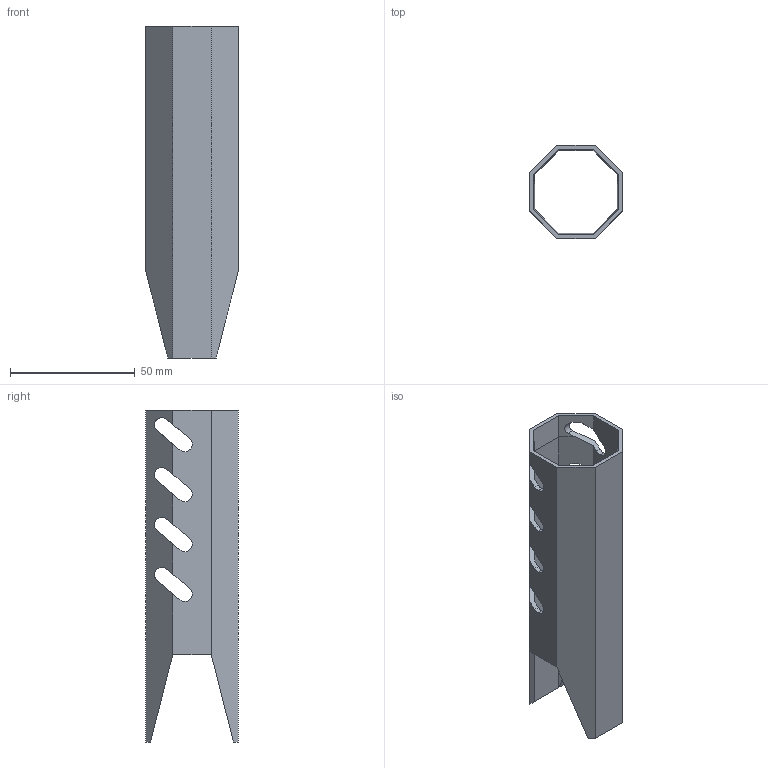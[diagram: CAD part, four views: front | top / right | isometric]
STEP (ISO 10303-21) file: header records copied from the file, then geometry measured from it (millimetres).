
FILE_DESCRIPTION (( 'STEP AP214' ), '1' );
FILE_NAME ('Handguard_Front.step', '2019-12-18T03:07:52', ( '' ), ( '' ), 'SwSTEP 2.0', 'SolidWorks 2019', '' );
FILE_SCHEMA (( 'AUTOMOTIVE_DESIGN' ));
Length unit declared in the file: millimetre
Products named in the file (1): Handguard_Front
Bounding box: 37.15 x 37.15 x 133 mm (x, y, z)
Volume: 24806.3 mm3; surface area: 26628.7 mm2
Topology: 1 solids, 1 shells, 73 faces, 250 edges, 162 vertices
Faces by surface type: plane 49, cylinder 24
Entity records: 2734 total; most frequent: CARTESIAN_POINT 534, ORIENTED_EDGE 500, DIRECTION 414, EDGE_CURVE 250, VECTOR 202, LINE 202, VERTEX_POINT 162, AXIS2_PLACEMENT_3D 106
